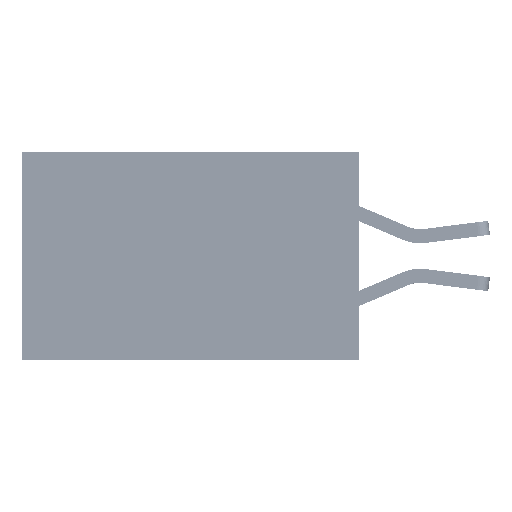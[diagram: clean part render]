
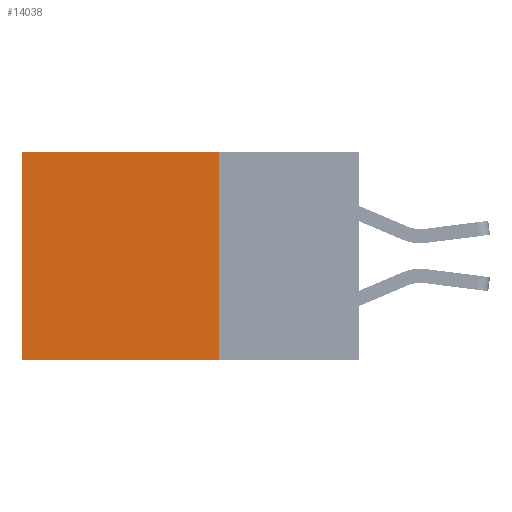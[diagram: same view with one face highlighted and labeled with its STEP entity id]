
A CAD part, left-side view. The second image highlights one B-rep face of the part: STEP entity #14038.
In plain terms, the highlighted planar face has unit normal (-1, 0, 0).
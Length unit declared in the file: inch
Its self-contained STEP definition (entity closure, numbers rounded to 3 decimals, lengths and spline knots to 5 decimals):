
#363 = CARTESIAN_POINT ( 'NONE',  ( 0.2875, 0.25, -0.37 ) ) ;
#513 = CARTESIAN_POINT ( 'NONE',  ( 0.2875, 0.6, -0.37 ) ) ;
#2469 = CARTESIAN_POINT ( 'NONE',  ( 0.2875, 0.6, 0. ) ) ;
#3803 = PLANE ( 'NONE',  #37291 ) ;
#5327 = LINE ( 'NONE', #32433, #12302 ) ;
#6941 = CARTESIAN_POINT ( 'NONE',  ( 0.2875, 0.25, 0. ) ) ;
#7212 = DIRECTION ( 'NONE',  ( 1., 0., 0. ) ) ;
#7842 = EDGE_CURVE ( 'NONE', #26536, #14343, #19338, .T. ) ;
#11859 = VECTOR ( 'NONE', #30579, 39.37008 ) ;
#12204 = DIRECTION ( 'NONE',  ( 0., 1., 0. ) ) ;
#12302 = VECTOR ( 'NONE', #20386, 39.37008 ) ;
#14038 = ADVANCED_FACE ( 'NONE', ( #36980 ), #3803, .F. ) ;
#14343 = VERTEX_POINT ( 'NONE', #23635 ) ;
#14435 = EDGE_CURVE ( 'NONE', #17343, #18682, #5327, .T. ) ;
#14566 = EDGE_LOOP ( 'NONE', ( #35602, #34462, #17747, #16485 ) ) ;
#15213 = VECTOR ( 'NONE', #12204, 39.37008 ) ;
#16140 = LINE ( 'NONE', #363, #15213 ) ;
#16485 = ORIENTED_EDGE ( 'NONE', *, *, #32408, .T. ) ;
#17343 = VERTEX_POINT ( 'NONE', #2469 ) ;
#17747 = ORIENTED_EDGE ( 'NONE', *, *, #7842, .F. ) ;
#18682 = VERTEX_POINT ( 'NONE', #513 ) ;
#18798 = CARTESIAN_POINT ( 'NONE',  ( 0.2875, 0.25, 0. ) ) ;
#19182 = DIRECTION ( 'NONE',  ( 0., 0., -1. ) ) ;
#19338 = LINE ( 'NONE', #27753, #11859 ) ;
#20386 = DIRECTION ( 'NONE',  ( 0., 0., -1. ) ) ;
#21715 = CARTESIAN_POINT ( 'NONE',  ( 0.2875, 0.25, 0. ) ) ;
#23635 = CARTESIAN_POINT ( 'NONE',  ( 0.2875, 0.25, -0.37 ) ) ;
#26152 = LINE ( 'NONE', #21715, #34922 ) ;
#26536 = VERTEX_POINT ( 'NONE', #6941 ) ;
#27753 = CARTESIAN_POINT ( 'NONE',  ( 0.2875, 0.25, 0. ) ) ;
#30579 = DIRECTION ( 'NONE',  ( 0., 0., -1. ) ) ;
#32408 = EDGE_CURVE ( 'NONE', #26536, #17343, #26152, .T. ) ;
#32433 = CARTESIAN_POINT ( 'NONE',  ( 0.2875, 0.6, 0. ) ) ;
#34462 = ORIENTED_EDGE ( 'NONE', *, *, #36822, .F. ) ;
#34922 = VECTOR ( 'NONE', #36354, 39.37008 ) ;
#35602 = ORIENTED_EDGE ( 'NONE', *, *, #14435, .T. ) ;
#36354 = DIRECTION ( 'NONE',  ( 0., 1., 0. ) ) ;
#36822 = EDGE_CURVE ( 'NONE', #14343, #18682, #16140, .T. ) ;
#36980 = FACE_OUTER_BOUND ( 'NONE', #14566, .T. ) ;
#37291 = AXIS2_PLACEMENT_3D ( 'NONE', #18798, #7212, #19182 ) ;
